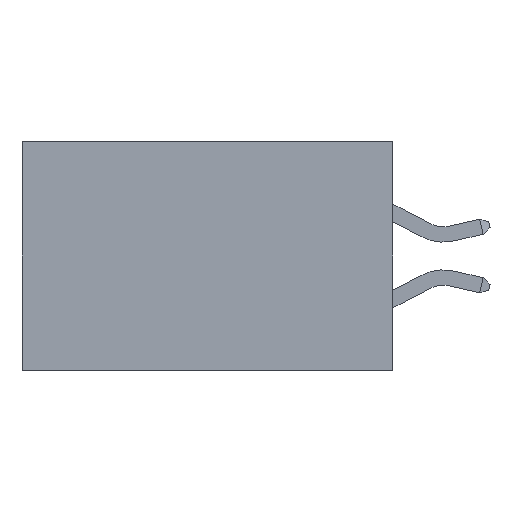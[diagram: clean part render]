
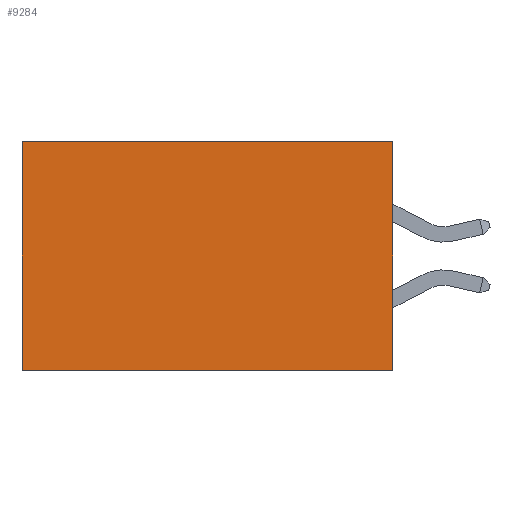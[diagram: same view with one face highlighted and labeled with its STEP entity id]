
A CAD part, left-side view. The second image highlights one B-rep face of the part: STEP entity #9284.
In plain terms, the highlighted planar face has unit normal (-1, 0, 0).
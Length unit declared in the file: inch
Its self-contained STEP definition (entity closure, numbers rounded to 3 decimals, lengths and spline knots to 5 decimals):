
#1614 = VECTOR ( 'NONE', #16902, 39.37008 ) ;
#2785 = EDGE_LOOP ( 'NONE', ( #22882, #20173, #10439, #3692 ) ) ;
#3692 = ORIENTED_EDGE ( 'NONE', *, *, #14255, .T. ) ;
#4303 = DIRECTION ( 'NONE',  ( 0., 0., -1. ) ) ;
#4892 = CARTESIAN_POINT ( 'NONE',  ( 0.2875, 0., -0.37 ) ) ;
#5301 = CARTESIAN_POINT ( 'NONE',  ( 0.2875, 0., 0. ) ) ;
#6730 = EDGE_CURVE ( 'NONE', #7277, #14696, #17453, .T. ) ;
#6823 = DIRECTION ( 'NONE',  ( 0., 1., 0. ) ) ;
#7052 = VECTOR ( 'NONE', #6823, 39.37008 ) ;
#7277 = VERTEX_POINT ( 'NONE', #10308 ) ;
#7674 = LINE ( 'NONE', #12953, #13501 ) ;
#8588 = CARTESIAN_POINT ( 'NONE',  ( 0.2875, 0.6, 0. ) ) ;
#8950 = PLANE ( 'NONE',  #18641 ) ;
#9284 = ADVANCED_FACE ( 'NONE', ( #13776 ), #8950, .F. ) ;
#10308 = CARTESIAN_POINT ( 'NONE',  ( 0.2875, 0., -0.37 ) ) ;
#10439 = ORIENTED_EDGE ( 'NONE', *, *, #14220, .F. ) ;
#10892 = DIRECTION ( 'NONE',  ( 1., 0., 0. ) ) ;
#11059 = LINE ( 'NONE', #15977, #20801 ) ;
#12700 = VERTEX_POINT ( 'NONE', #8588 ) ;
#12953 = CARTESIAN_POINT ( 'NONE',  ( 0.2875, 0., 0. ) ) ;
#13501 = VECTOR ( 'NONE', #24420, 39.37008 ) ;
#13776 = FACE_OUTER_BOUND ( 'NONE', #2785, .T. ) ;
#13913 = EDGE_CURVE ( 'NONE', #12700, #14696, #11059, .T. ) ;
#14029 = VERTEX_POINT ( 'NONE', #20107 ) ;
#14220 = EDGE_CURVE ( 'NONE', #14029, #7277, #7674, .T. ) ;
#14255 = EDGE_CURVE ( 'NONE', #14029, #12700, #22300, .T. ) ;
#14696 = VERTEX_POINT ( 'NONE', #18587 ) ;
#15977 = CARTESIAN_POINT ( 'NONE',  ( 0.2875, 0.6, 0. ) ) ;
#16902 = DIRECTION ( 'NONE',  ( 0., 1., 0. ) ) ;
#17453 = LINE ( 'NONE', #4892, #7052 ) ;
#18587 = CARTESIAN_POINT ( 'NONE',  ( 0.2875, 0.6, -0.37 ) ) ;
#18641 = AXIS2_PLACEMENT_3D ( 'NONE', #22519, #10892, #24409 ) ;
#20107 = CARTESIAN_POINT ( 'NONE',  ( 0.2875, 0., 0. ) ) ;
#20173 = ORIENTED_EDGE ( 'NONE', *, *, #6730, .F. ) ;
#20801 = VECTOR ( 'NONE', #4303, 39.37008 ) ;
#22300 = LINE ( 'NONE', #5301, #1614 ) ;
#22519 = CARTESIAN_POINT ( 'NONE',  ( 0.2875, 0., 0. ) ) ;
#22882 = ORIENTED_EDGE ( 'NONE', *, *, #13913, .T. ) ;
#24409 = DIRECTION ( 'NONE',  ( 0., 0., -1. ) ) ;
#24420 = DIRECTION ( 'NONE',  ( 0., 0., -1. ) ) ;
